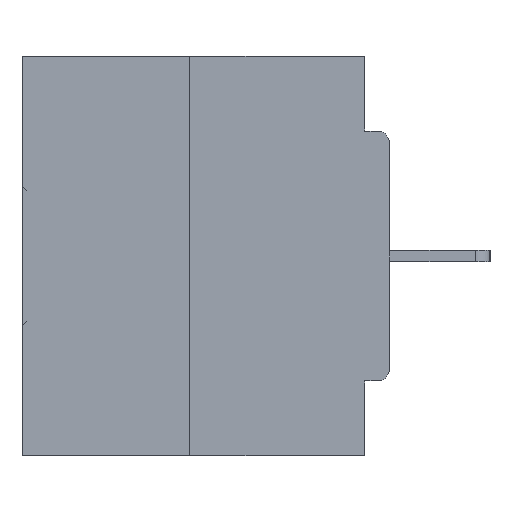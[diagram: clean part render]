
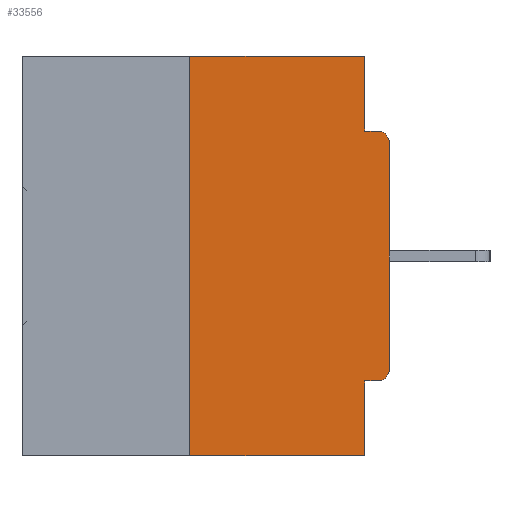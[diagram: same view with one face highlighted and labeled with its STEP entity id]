
A CAD part, left-side view. The second image highlights one B-rep face of the part: STEP entity #33556.
In plain terms, the highlighted planar face has unit normal (-1, 0, 0).
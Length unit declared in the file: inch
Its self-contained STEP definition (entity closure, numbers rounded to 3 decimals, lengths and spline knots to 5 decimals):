
#344 = DIRECTION ( 'NONE',  ( 1., 0., 0. ) ) ;
#944 = DIRECTION ( 'NONE',  ( 0., 0., -1. ) ) ;
#1157 = DIRECTION ( 'NONE',  ( 0., 0., 1. ) ) ;
#1257 = LINE ( 'NONE', #12155, #16398 ) ;
#1999 = CARTESIAN_POINT ( 'NONE',  ( 0., 0., -0.0935 ) ) ;
#2112 = DIRECTION ( 'NONE',  ( 0., -1., 0. ) ) ;
#2228 = AXIS2_PLACEMENT_3D ( 'NONE', #35345, #17613, #38261 ) ;
#2319 = VERTEX_POINT ( 'NONE', #23041 ) ;
#3109 = VERTEX_POINT ( 'NONE', #35880 ) ;
#4618 = EDGE_CURVE ( 'NONE', #35194, #19959, #12718, .T. ) ;
#4716 = ORIENTED_EDGE ( 'NONE', *, *, #27953, .F. ) ;
#5094 = DIRECTION ( 'NONE',  ( 0., -1., 0. ) ) ;
#5297 = DIRECTION ( 'NONE',  ( 0., 0., 1. ) ) ;
#6007 = FACE_OUTER_BOUND ( 'NONE', #35280, .T. ) ;
#6916 = LINE ( 'NONE', #19029, #37574 ) ;
#7469 = LINE ( 'NONE', #1999, #16362 ) ;
#7602 = DIRECTION ( 'NONE',  ( -1., 0., 0. ) ) ;
#8613 = LINE ( 'NONE', #37822, #23490 ) ;
#9299 = AXIS2_PLACEMENT_3D ( 'NONE', #36170, #344, #21419 ) ;
#10914 = ORIENTED_EDGE ( 'NONE', *, *, #33263, .F. ) ;
#11173 = VECTOR ( 'NONE', #1157, 39.37008 ) ;
#11218 = CARTESIAN_POINT ( 'NONE',  ( 0., 0.031, -0.5 ) ) ;
#11304 = LINE ( 'NONE', #32068, #26146 ) ;
#11374 = ORIENTED_EDGE ( 'NONE', *, *, #36511, .F. ) ;
#11884 = VECTOR ( 'NONE', #14184, 39.37008 ) ;
#12099 = LINE ( 'NONE', #16373, #11173 ) ;
#12155 = CARTESIAN_POINT ( 'NONE',  ( 0., 0.46, -0.5 ) ) ;
#12304 = VERTEX_POINT ( 'NONE', #34570 ) ;
#12718 = CIRCLE ( 'NONE', #12949, 0.015 ) ;
#12820 = EDGE_CURVE ( 'NONE', #19959, #24114, #12099, .T. ) ;
#12949 = AXIS2_PLACEMENT_3D ( 'NONE', #25432, #7602, #28454 ) ;
#13651 = CARTESIAN_POINT ( 'NONE',  ( 0., 0., -0.3915 ) ) ;
#13743 = CIRCLE ( 'NONE', #2228, 0.015 ) ;
#14184 = DIRECTION ( 'NONE',  ( 0., 0., -1. ) ) ;
#15124 = DIRECTION ( 'NONE',  ( 0., -1., 0. ) ) ;
#15341 = EDGE_CURVE ( 'NONE', #24114, #2319, #13743, .T. ) ;
#15517 = VERTEX_POINT ( 'NONE', #30076 ) ;
#15996 = ORIENTED_EDGE ( 'NONE', *, *, #15341, .T. ) ;
#16362 = VECTOR ( 'NONE', #5094, 39.37008 ) ;
#16373 = CARTESIAN_POINT ( 'NONE',  ( 0., 0., 0. ) ) ;
#16398 = VECTOR ( 'NONE', #15124, 39.37008 ) ;
#16466 = ORIENTED_EDGE ( 'NONE', *, *, #37003, .F. ) ;
#17153 = CARTESIAN_POINT ( 'NONE',  ( 0., 0.031, -0.5 ) ) ;
#17613 = DIRECTION ( 'NONE',  ( -1., 0., 0. ) ) ;
#18320 = ORIENTED_EDGE ( 'NONE', *, *, #32783, .T. ) ;
#19029 = CARTESIAN_POINT ( 'NONE',  ( 0., 0.031, 0. ) ) ;
#19959 = VERTEX_POINT ( 'NONE', #13651 ) ;
#20531 = CARTESIAN_POINT ( 'NONE',  ( 0., 0., -0.4065 ) ) ;
#21100 = ORIENTED_EDGE ( 'NONE', *, *, #4618, .T. ) ;
#21419 = DIRECTION ( 'NONE',  ( 0., 0., -1. ) ) ;
#23041 = CARTESIAN_POINT ( 'NONE',  ( 0., 0.015, -0.0935 ) ) ;
#23490 = VECTOR ( 'NONE', #2112, 39.37008 ) ;
#24114 = VERTEX_POINT ( 'NONE', #29094 ) ;
#25432 = CARTESIAN_POINT ( 'NONE',  ( 0., 0.015, -0.3915 ) ) ;
#26146 = VECTOR ( 'NONE', #5297, 39.37008 ) ;
#27953 = EDGE_CURVE ( 'NONE', #3109, #12304, #6916, .T. ) ;
#28454 = DIRECTION ( 'NONE',  ( 0., 0., -1. ) ) ;
#29094 = CARTESIAN_POINT ( 'NONE',  ( 0., 0., -0.1085 ) ) ;
#29156 = VERTEX_POINT ( 'NONE', #30234 ) ;
#29218 = VERTEX_POINT ( 'NONE', #30609 ) ;
#30076 = CARTESIAN_POINT ( 'NONE',  ( 0., 0.25, 0. ) ) ;
#30234 = CARTESIAN_POINT ( 'NONE',  ( 0., 0.031, -0.4065 ) ) ;
#30609 = CARTESIAN_POINT ( 'NONE',  ( 0., 0.25, -0.5 ) ) ;
#30901 = ORIENTED_EDGE ( 'NONE', *, *, #12820, .T. ) ;
#31857 = VECTOR ( 'NONE', #38224, 39.37008 ) ;
#32068 = CARTESIAN_POINT ( 'NONE',  ( 0., 0.25, 0. ) ) ;
#32783 = EDGE_CURVE ( 'NONE', #29218, #35162, #1257, .T. ) ;
#33191 = ORIENTED_EDGE ( 'NONE', *, *, #38568, .F. ) ;
#33250 = PLANE ( 'NONE',  #9299 ) ;
#33263 = EDGE_CURVE ( 'NONE', #12304, #2319, #7469, .T. ) ;
#33556 = ADVANCED_FACE ( 'NONE', ( #6007 ), #33250, .F. ) ;
#34570 = CARTESIAN_POINT ( 'NONE',  ( 0., 0.031, -0.0935 ) ) ;
#34616 = LINE ( 'NONE', #11218, #11884 ) ;
#35013 = CARTESIAN_POINT ( 'NONE',  ( 0., 0.015, -0.4065 ) ) ;
#35162 = VERTEX_POINT ( 'NONE', #17153 ) ;
#35194 = VERTEX_POINT ( 'NONE', #35013 ) ;
#35280 = EDGE_LOOP ( 'NONE', ( #16466, #33191, #18320, #11374, #35916, #21100, #30901, #15996, #10914, #4716 ) ) ;
#35345 = CARTESIAN_POINT ( 'NONE',  ( 0., 0.015, -0.1085 ) ) ;
#35880 = CARTESIAN_POINT ( 'NONE',  ( 0., 0.031, 0. ) ) ;
#35916 = ORIENTED_EDGE ( 'NONE', *, *, #36605, .F. ) ;
#36170 = CARTESIAN_POINT ( 'NONE',  ( 0., 0.46, 0. ) ) ;
#36511 = EDGE_CURVE ( 'NONE', #29156, #35162, #34616, .T. ) ;
#36605 = EDGE_CURVE ( 'NONE', #35194, #29156, #38698, .T. ) ;
#37003 = EDGE_CURVE ( 'NONE', #15517, #3109, #8613, .T. ) ;
#37574 = VECTOR ( 'NONE', #944, 39.37008 ) ;
#37822 = CARTESIAN_POINT ( 'NONE',  ( 0., 0.46, 0. ) ) ;
#38224 = DIRECTION ( 'NONE',  ( 0., 1., 0. ) ) ;
#38261 = DIRECTION ( 'NONE',  ( 0., 0., -1. ) ) ;
#38568 = EDGE_CURVE ( 'NONE', #29218, #15517, #11304, .T. ) ;
#38698 = LINE ( 'NONE', #20531, #31857 ) ;
